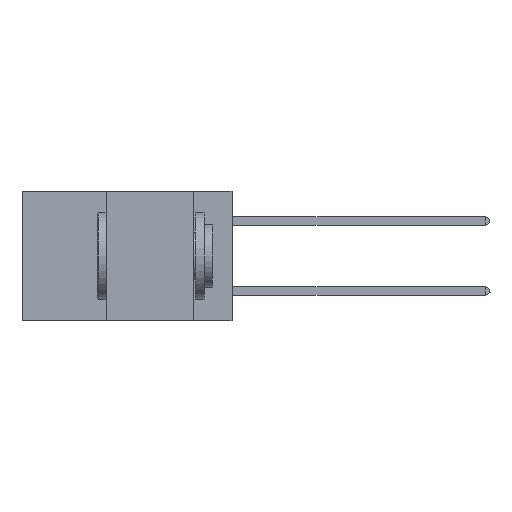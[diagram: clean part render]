
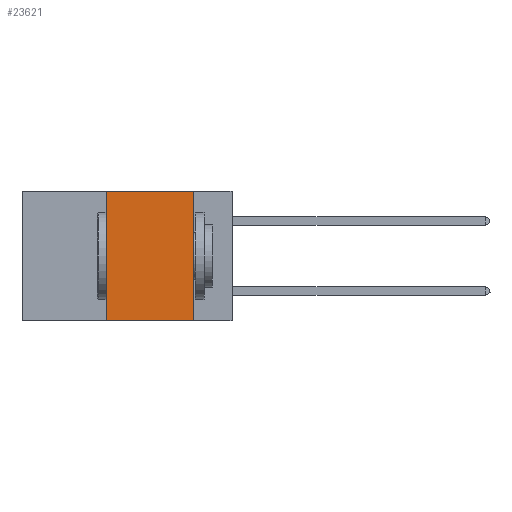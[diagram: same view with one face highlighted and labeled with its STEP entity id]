
A CAD part, left-side view. The second image highlights one B-rep face of the part: STEP entity #23621.
In plain terms, the highlighted planar face has unit normal (-1, 0, 0).
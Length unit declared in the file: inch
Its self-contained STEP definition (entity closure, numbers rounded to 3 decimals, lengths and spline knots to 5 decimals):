
#91 = DIRECTION ( 'NONE',  ( 0., 0., -1. ) ) ;
#1356 = CARTESIAN_POINT ( 'NONE',  ( 0., 0.36, 0. ) ) ;
#1542 = DIRECTION ( 'NONE',  ( 0., -1., 0. ) ) ;
#2145 = DIRECTION ( 'NONE',  ( 0., 0., -1. ) ) ;
#2758 = EDGE_CURVE ( 'NONE', #25446, #9692, #15010, .T. ) ;
#3287 = EDGE_CURVE ( 'NONE', #9900, #25446, #4961, .T. ) ;
#3432 = EDGE_CURVE ( 'NONE', #21844, #9900, #16233, .T. ) ;
#3641 = VECTOR ( 'NONE', #1542, 39.37008 ) ;
#3948 = DIRECTION ( 'NONE',  ( 1., 0., 0. ) ) ;
#4961 = LINE ( 'NONE', #22105, #9620 ) ;
#5519 = CARTESIAN_POINT ( 'NONE',  ( 0., 0.11, -0.37 ) ) ;
#5572 = CARTESIAN_POINT ( 'NONE',  ( 0., 0.6, -0.37 ) ) ;
#8013 = ORIENTED_EDGE ( 'NONE', *, *, #3432, .F. ) ;
#8406 = VECTOR ( 'NONE', #2145, 39.37008 ) ;
#9620 = VECTOR ( 'NONE', #22186, 39.37008 ) ;
#9692 = VERTEX_POINT ( 'NONE', #5519 ) ;
#9900 = VERTEX_POINT ( 'NONE', #1356 ) ;
#11470 = LINE ( 'NONE', #5572, #3641 ) ;
#11542 = FACE_OUTER_BOUND ( 'NONE', #12417, .T. ) ;
#11960 = CARTESIAN_POINT ( 'NONE',  ( 0., 0.11, 0. ) ) ;
#12187 = ORIENTED_EDGE ( 'NONE', *, *, #3287, .F. ) ;
#12417 = EDGE_LOOP ( 'NONE', ( #13996, #12187, #8013, #12574 ) ) ;
#12574 = ORIENTED_EDGE ( 'NONE', *, *, #24610, .T. ) ;
#13996 = ORIENTED_EDGE ( 'NONE', *, *, #2758, .F. ) ;
#15010 = LINE ( 'NONE', #11960, #8406 ) ;
#15838 = CARTESIAN_POINT ( 'NONE',  ( 0., 0.36, -0.37 ) ) ;
#16233 = LINE ( 'NONE', #19741, #20333 ) ;
#17511 = DIRECTION ( 'NONE',  ( 0., 0., 1. ) ) ;
#18520 = CARTESIAN_POINT ( 'NONE',  ( 0., 0.11, 0. ) ) ;
#18951 = AXIS2_PLACEMENT_3D ( 'NONE', #24033, #3948, #91 ) ;
#19741 = CARTESIAN_POINT ( 'NONE',  ( 0., 0.36, 0. ) ) ;
#20035 = PLANE ( 'NONE',  #18951 ) ;
#20333 = VECTOR ( 'NONE', #17511, 39.37008 ) ;
#21844 = VERTEX_POINT ( 'NONE', #15838 ) ;
#22105 = CARTESIAN_POINT ( 'NONE',  ( 0., 0.6, 0. ) ) ;
#22186 = DIRECTION ( 'NONE',  ( 0., -1., 0. ) ) ;
#23621 = ADVANCED_FACE ( 'NONE', ( #11542 ), #20035, .F. ) ;
#24033 = CARTESIAN_POINT ( 'NONE',  ( 0., 0.6, 0. ) ) ;
#24610 = EDGE_CURVE ( 'NONE', #21844, #9692, #11470, .T. ) ;
#25446 = VERTEX_POINT ( 'NONE', #18520 ) ;
